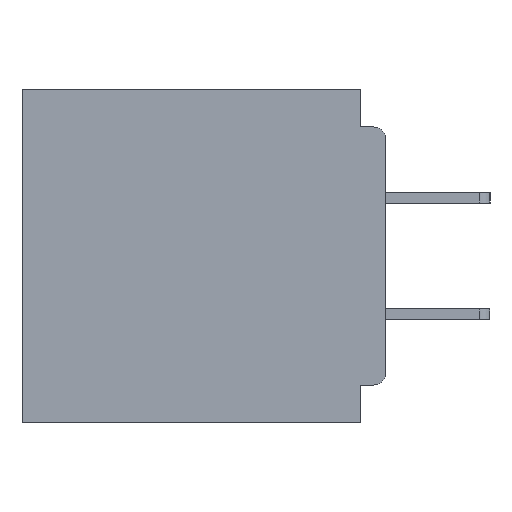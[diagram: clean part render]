
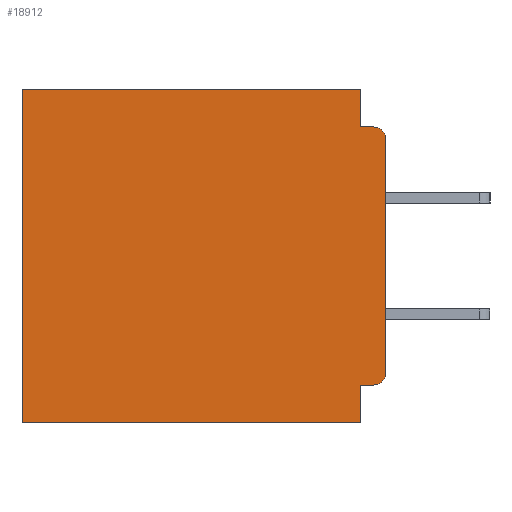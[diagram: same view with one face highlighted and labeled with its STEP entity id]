
A CAD part, left-side view. The second image highlights one B-rep face of the part: STEP entity #18912.
In plain terms, the highlighted planar face has unit normal (-1, 0, 0).
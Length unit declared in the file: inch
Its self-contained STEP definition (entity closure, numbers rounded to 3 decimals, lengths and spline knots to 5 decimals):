
#339 = VERTEX_POINT ( 'NONE', #5842 ) ;
#738 = LINE ( 'NONE', #4606, #22039 ) ;
#785 = CARTESIAN_POINT ( 'NONE',  ( 0.3, 0.437, -0.4 ) ) ;
#1031 = CARTESIAN_POINT ( 'NONE',  ( 0.3, 0.437, -0.4 ) ) ;
#1177 = VERTEX_POINT ( 'NONE', #34130 ) ;
#1254 = CARTESIAN_POINT ( 'NONE',  ( 0.3, 0.031, -0.4 ) ) ;
#1675 = CIRCLE ( 'NONE', #35474, 0.015 ) ;
#1952 = LINE ( 'NONE', #2658, #23234 ) ;
#2161 = DIRECTION ( 'NONE',  ( 0., 0., -1. ) ) ;
#2370 = VERTEX_POINT ( 'NONE', #9722 ) ;
#2658 = CARTESIAN_POINT ( 'NONE',  ( 0.3, 0., -0.4 ) ) ;
#4065 = LINE ( 'NONE', #9235, #26327 ) ;
#4185 = ORIENTED_EDGE ( 'NONE', *, *, #15545, .F. ) ;
#4224 = DIRECTION ( 'NONE',  ( -1., 0., 0. ) ) ;
#4364 = ORIENTED_EDGE ( 'NONE', *, *, #4561, .T. ) ;
#4561 = EDGE_CURVE ( 'NONE', #28611, #2370, #23777, .T. ) ;
#4606 = CARTESIAN_POINT ( 'NONE',  ( 0.3, 0.031, 0. ) ) ;
#4783 = CARTESIAN_POINT ( 'NONE',  ( 0.3, 0.031, 0. ) ) ;
#5125 = VERTEX_POINT ( 'NONE', #1031 ) ;
#5842 = CARTESIAN_POINT ( 'NONE',  ( 0.3, 0.015, -0.355 ) ) ;
#6052 = ORIENTED_EDGE ( 'NONE', *, *, #20939, .F. ) ;
#6465 = ORIENTED_EDGE ( 'NONE', *, *, #17901, .F. ) ;
#6490 = VERTEX_POINT ( 'NONE', #21832 ) ;
#6794 = LINE ( 'NONE', #7704, #29085 ) ;
#6899 = VERTEX_POINT ( 'NONE', #1254 ) ;
#7704 = CARTESIAN_POINT ( 'NONE',  ( 0.3, 0., -0.355 ) ) ;
#8161 = EDGE_CURVE ( 'NONE', #339, #1177, #6794, .T. ) ;
#8308 = DIRECTION ( 'NONE',  ( 0., 0., -1. ) ) ;
#9235 = CARTESIAN_POINT ( 'NONE',  ( 0.3, 0., -0.4 ) ) ;
#9722 = CARTESIAN_POINT ( 'NONE',  ( 0.3, 0.437, 0. ) ) ;
#10152 = CARTESIAN_POINT ( 'NONE',  ( 0.3, 0., 0. ) ) ;
#10445 = ORIENTED_EDGE ( 'NONE', *, *, #22359, .T. ) ;
#10544 = CARTESIAN_POINT ( 'NONE',  ( 0.3, 0.031, -0.4 ) ) ;
#10658 = DIRECTION ( 'NONE',  ( 0., 1., 0. ) ) ;
#13267 = VECTOR ( 'NONE', #24937, 39.37008 ) ;
#13412 = DIRECTION ( 'NONE',  ( 0., 0., -1. ) ) ;
#14853 = LINE ( 'NONE', #785, #21586 ) ;
#15290 = CARTESIAN_POINT ( 'NONE',  ( 0.3, 0., -0.34 ) ) ;
#15545 = EDGE_CURVE ( 'NONE', #1177, #6899, #20857, .T. ) ;
#17140 = VERTEX_POINT ( 'NONE', #18289 ) ;
#17733 = EDGE_CURVE ( 'NONE', #2370, #5125, #14853, .T. ) ;
#17901 = EDGE_CURVE ( 'NONE', #28611, #6490, #738, .T. ) ;
#17913 = ORIENTED_EDGE ( 'NONE', *, *, #17733, .T. ) ;
#18289 = CARTESIAN_POINT ( 'NONE',  ( 0.3, 0., -0.06 ) ) ;
#18912 = ADVANCED_FACE ( 'NONE', ( #32572 ), #22691, .F. ) ;
#19502 = DIRECTION ( 'NONE',  ( -1., 0., 0. ) ) ;
#20857 = LINE ( 'NONE', #10544, #13267 ) ;
#20939 = EDGE_CURVE ( 'NONE', #6899, #5125, #1952, .T. ) ;
#21530 = CARTESIAN_POINT ( 'NONE',  ( 0.3, 0.015, -0.06 ) ) ;
#21586 = VECTOR ( 'NONE', #23984, 39.37008 ) ;
#21633 = VERTEX_POINT ( 'NONE', #15290 ) ;
#21832 = CARTESIAN_POINT ( 'NONE',  ( 0.3, 0.031, -0.045 ) ) ;
#22039 = VECTOR ( 'NONE', #13412, 39.37008 ) ;
#22359 = EDGE_CURVE ( 'NONE', #17140, #22897, #32222, .T. ) ;
#22462 = ORIENTED_EDGE ( 'NONE', *, *, #35893, .F. ) ;
#22691 = PLANE ( 'NONE',  #35862 ) ;
#22897 = VERTEX_POINT ( 'NONE', #36089 ) ;
#23065 = EDGE_LOOP ( 'NONE', ( #22462, #10445, #33687, #6465, #4364, #17913, #6052, #4185, #31068, #35541 ) ) ;
#23085 = EDGE_CURVE ( 'NONE', #339, #21633, #1675, .T. ) ;
#23220 = AXIS2_PLACEMENT_3D ( 'NONE', #21530, #4224, #24512 ) ;
#23234 = VECTOR ( 'NONE', #34718, 39.37008 ) ;
#23777 = LINE ( 'NONE', #10152, #32507 ) ;
#23984 = DIRECTION ( 'NONE',  ( 0., 0., -1. ) ) ;
#24512 = DIRECTION ( 'NONE',  ( 0., 0., -1. ) ) ;
#24887 = EDGE_CURVE ( 'NONE', #6490, #22897, #37458, .T. ) ;
#24937 = DIRECTION ( 'NONE',  ( 0., 0., -1. ) ) ;
#25638 = DIRECTION ( 'NONE',  ( 1., 0., 0. ) ) ;
#25975 = DIRECTION ( 'NONE',  ( 0., -1., 0. ) ) ;
#26327 = VECTOR ( 'NONE', #29517, 39.37008 ) ;
#28611 = VERTEX_POINT ( 'NONE', #4783 ) ;
#29085 = VECTOR ( 'NONE', #10658, 39.37008 ) ;
#29517 = DIRECTION ( 'NONE',  ( 0., 0., -1. ) ) ;
#29700 = VECTOR ( 'NONE', #25975, 39.37008 ) ;
#30433 = DIRECTION ( 'NONE',  ( 0., 1., 0. ) ) ;
#31068 = ORIENTED_EDGE ( 'NONE', *, *, #8161, .F. ) ;
#31410 = CARTESIAN_POINT ( 'NONE',  ( 0.3, 0., -0.4 ) ) ;
#31743 = CARTESIAN_POINT ( 'NONE',  ( 0.3, 0., -0.045 ) ) ;
#32222 = CIRCLE ( 'NONE', #23220, 0.015 ) ;
#32507 = VECTOR ( 'NONE', #30433, 39.37008 ) ;
#32572 = FACE_OUTER_BOUND ( 'NONE', #23065, .T. ) ;
#33687 = ORIENTED_EDGE ( 'NONE', *, *, #24887, .F. ) ;
#34130 = CARTESIAN_POINT ( 'NONE',  ( 0.3, 0.031, -0.355 ) ) ;
#34718 = DIRECTION ( 'NONE',  ( 0., 1., 0. ) ) ;
#35474 = AXIS2_PLACEMENT_3D ( 'NONE', #36982, #19502, #2161 ) ;
#35541 = ORIENTED_EDGE ( 'NONE', *, *, #23085, .T. ) ;
#35862 = AXIS2_PLACEMENT_3D ( 'NONE', #31410, #25638, #8308 ) ;
#35893 = EDGE_CURVE ( 'NONE', #17140, #21633, #4065, .T. ) ;
#36089 = CARTESIAN_POINT ( 'NONE',  ( 0.3, 0.015, -0.045 ) ) ;
#36982 = CARTESIAN_POINT ( 'NONE',  ( 0.3, 0.015, -0.34 ) ) ;
#37458 = LINE ( 'NONE', #31743, #29700 ) ;
